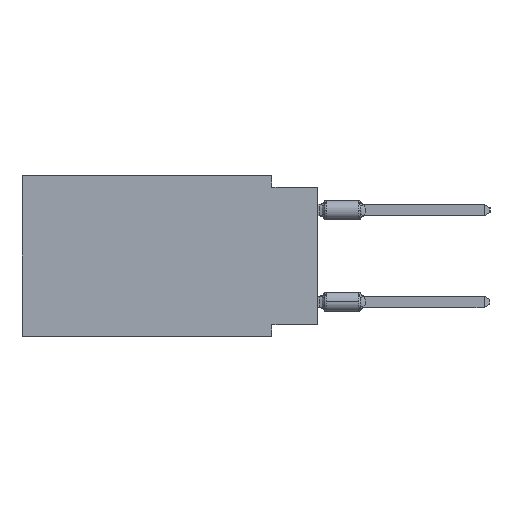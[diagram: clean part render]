
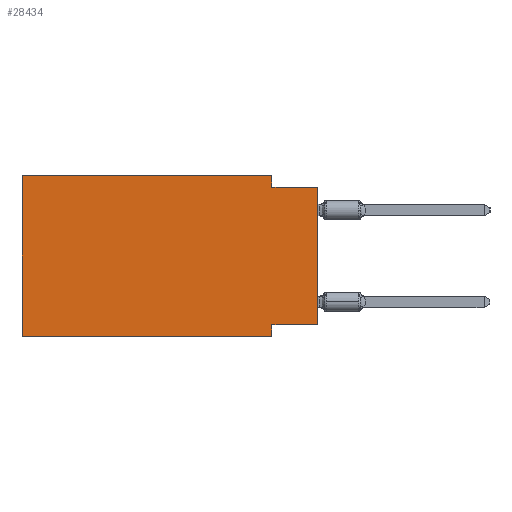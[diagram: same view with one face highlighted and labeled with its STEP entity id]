
A CAD part, left-side view. The second image highlights one B-rep face of the part: STEP entity #28434.
In plain terms, the highlighted planar face has unit normal (-1, 0, 0).
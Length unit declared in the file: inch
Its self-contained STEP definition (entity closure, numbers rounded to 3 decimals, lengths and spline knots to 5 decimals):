
#87 = VECTOR ( 'NONE', #3224, 39.37008 ) ;
#486 = ORIENTED_EDGE ( 'NONE', *, *, #3652, .F. ) ;
#721 = VECTOR ( 'NONE', #28374, 39.37008 ) ;
#1195 = ORIENTED_EDGE ( 'NONE', *, *, #21230, .F. ) ;
#1728 = ORIENTED_EDGE ( 'NONE', *, *, #17545, .F. ) ;
#1754 = VERTEX_POINT ( 'NONE', #9020 ) ;
#2216 = AXIS2_PLACEMENT_3D ( 'NONE', #10255, #19196, #21262 ) ;
#2632 = CARTESIAN_POINT ( 'NONE',  ( 0., 0.1, 0. ) ) ;
#3146 = EDGE_CURVE ( 'NONE', #1754, #4465, #15141, .T. ) ;
#3224 = DIRECTION ( 'NONE',  ( 0., -1., 0. ) ) ;
#3652 = EDGE_CURVE ( 'NONE', #25343, #1754, #24905, .T. ) ;
#3815 = CARTESIAN_POINT ( 'NONE',  ( 0., 0.1, -0.35 ) ) ;
#4465 = VERTEX_POINT ( 'NONE', #23497 ) ;
#4919 = LINE ( 'NONE', #13977, #22173 ) ;
#5155 = VECTOR ( 'NONE', #25735, 39.37008 ) ;
#5947 = CARTESIAN_POINT ( 'NONE',  ( 0., 0.645, 0. ) ) ;
#6978 = VERTEX_POINT ( 'NONE', #9663 ) ;
#7079 = CARTESIAN_POINT ( 'NONE',  ( 0., 0., 0. ) ) ;
#7092 = EDGE_CURVE ( 'NONE', #6978, #11970, #16687, .T. ) ;
#8490 = CARTESIAN_POINT ( 'NONE',  ( 0., 0.645, -0.35 ) ) ;
#8554 = CARTESIAN_POINT ( 'NONE',  ( 0., 0., -0.325 ) ) ;
#9020 = CARTESIAN_POINT ( 'NONE',  ( 0., 0.1, -0.325 ) ) ;
#9111 = CARTESIAN_POINT ( 'NONE',  ( 0., 0.1, -0.025 ) ) ;
#9203 = DIRECTION ( 'NONE',  ( 0., 0., -1. ) ) ;
#9663 = CARTESIAN_POINT ( 'NONE',  ( 0., 0.645, -0.35 ) ) ;
#9936 = LINE ( 'NONE', #23601, #87 ) ;
#10255 = CARTESIAN_POINT ( 'NONE',  ( 0., 0.645, 0. ) ) ;
#11870 = EDGE_CURVE ( 'NONE', #6978, #4465, #22170, .T. ) ;
#11970 = VERTEX_POINT ( 'NONE', #24699 ) ;
#13507 = ORIENTED_EDGE ( 'NONE', *, *, #28291, .F. ) ;
#13977 = CARTESIAN_POINT ( 'NONE',  ( 0., 0., -0.025 ) ) ;
#14015 = CARTESIAN_POINT ( 'NONE',  ( 0., 0.1, 0. ) ) ;
#14104 = FACE_OUTER_BOUND ( 'NONE', #15519, .T. ) ;
#14213 = LINE ( 'NONE', #7079, #14302 ) ;
#14302 = VECTOR ( 'NONE', #20927, 39.37008 ) ;
#14858 = ORIENTED_EDGE ( 'NONE', *, *, #7092, .F. ) ;
#15141 = LINE ( 'NONE', #3815, #721 ) ;
#15519 = EDGE_LOOP ( 'NONE', ( #21420, #13507, #1195, #1728, #14858, #22561, #24521, #486 ) ) ;
#16687 = LINE ( 'NONE', #5947, #5155 ) ;
#16825 = PLANE ( 'NONE',  #2216 ) ;
#17213 = VECTOR ( 'NONE', #29038, 39.37008 ) ;
#17545 = EDGE_CURVE ( 'NONE', #11970, #19625, #9936, .T. ) ;
#19196 = DIRECTION ( 'NONE',  ( 1., 0., 0. ) ) ;
#19625 = VERTEX_POINT ( 'NONE', #14015 ) ;
#19741 = VECTOR ( 'NONE', #26994, 39.37008 ) ;
#20826 = DIRECTION ( 'NONE',  ( 0., -1., 0. ) ) ;
#20927 = DIRECTION ( 'NONE',  ( 0., 0., 1. ) ) ;
#21230 = EDGE_CURVE ( 'NONE', #19625, #23928, #22707, .T. ) ;
#21262 = DIRECTION ( 'NONE',  ( 0., 0., -1. ) ) ;
#21420 = ORIENTED_EDGE ( 'NONE', *, *, #23774, .T. ) ;
#22170 = LINE ( 'NONE', #8490, #17213 ) ;
#22173 = VECTOR ( 'NONE', #20826, 39.37008 ) ;
#22191 = VERTEX_POINT ( 'NONE', #27531 ) ;
#22330 = CARTESIAN_POINT ( 'NONE',  ( 0., 0., -0.325 ) ) ;
#22561 = ORIENTED_EDGE ( 'NONE', *, *, #11870, .T. ) ;
#22707 = LINE ( 'NONE', #2632, #29412 ) ;
#23497 = CARTESIAN_POINT ( 'NONE',  ( 0., 0.1, -0.35 ) ) ;
#23601 = CARTESIAN_POINT ( 'NONE',  ( 0., 0.645, 0. ) ) ;
#23774 = EDGE_CURVE ( 'NONE', #25343, #22191, #14213, .T. ) ;
#23928 = VERTEX_POINT ( 'NONE', #9111 ) ;
#24521 = ORIENTED_EDGE ( 'NONE', *, *, #3146, .F. ) ;
#24699 = CARTESIAN_POINT ( 'NONE',  ( 0., 0.645, 0. ) ) ;
#24905 = LINE ( 'NONE', #8554, #19741 ) ;
#25343 = VERTEX_POINT ( 'NONE', #22330 ) ;
#25735 = DIRECTION ( 'NONE',  ( 0., 0., 1. ) ) ;
#26994 = DIRECTION ( 'NONE',  ( 0., 1., 0. ) ) ;
#27531 = CARTESIAN_POINT ( 'NONE',  ( 0., 0., -0.025 ) ) ;
#28291 = EDGE_CURVE ( 'NONE', #23928, #22191, #4919, .T. ) ;
#28374 = DIRECTION ( 'NONE',  ( 0., 0., -1. ) ) ;
#28434 = ADVANCED_FACE ( 'NONE', ( #14104 ), #16825, .F. ) ;
#29038 = DIRECTION ( 'NONE',  ( 0., -1., 0. ) ) ;
#29412 = VECTOR ( 'NONE', #9203, 39.37008 ) ;
